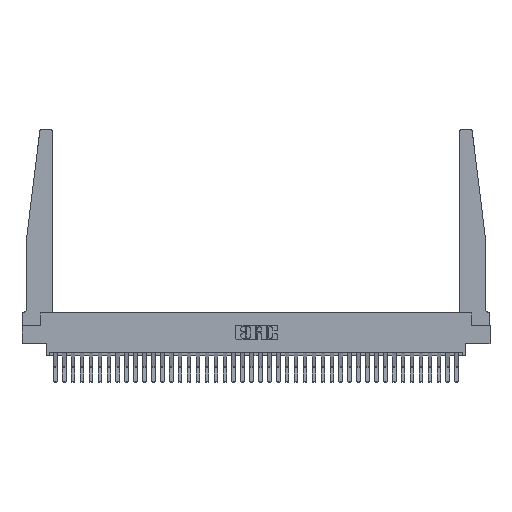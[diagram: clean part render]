
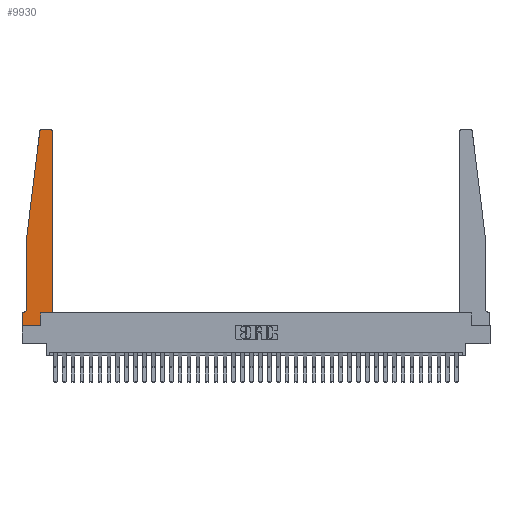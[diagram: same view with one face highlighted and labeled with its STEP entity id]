
A CAD part, top view. The second image highlights one B-rep face of the part: STEP entity #9930.
In plain terms, the highlighted planar face has unit normal (0, 0, 1).
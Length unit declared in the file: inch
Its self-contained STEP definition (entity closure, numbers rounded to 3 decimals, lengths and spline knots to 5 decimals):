
#721 = CARTESIAN_POINT ( 'NONE',  ( 0., 0., 0.37 ) ) ;
#744 = VECTOR ( 'NONE', #24177, 39.37008 ) ;
#1113 = CARTESIAN_POINT ( 'NONE',  ( 0.065, 1.25, 0.37 ) ) ;
#1154 = VERTEX_POINT ( 'NONE', #30985 ) ;
#1266 = AXIS2_PLACEMENT_3D ( 'NONE', #10810, #29415, #13551 ) ;
#1383 = VERTEX_POINT ( 'NONE', #18739 ) ;
#1935 = CARTESIAN_POINT ( 'NONE',  ( 0.425, 2.72, 0.37 ) ) ;
#2070 = CARTESIAN_POINT ( 'NONE',  ( 0.2605, 0.18, 0.37 ) ) ;
#2180 = LINE ( 'NONE', #16580, #28918 ) ;
#3547 = CARTESIAN_POINT ( 'NONE',  ( 0.065, 0.1875, 0.37 ) ) ;
#4044 = VERTEX_POINT ( 'NONE', #24911 ) ;
#4615 = LINE ( 'NONE', #6835, #32141 ) ;
#4649 = DIRECTION ( 'NONE',  ( 1., 0., 0. ) ) ;
#4755 = LINE ( 'NONE', #2070, #25186 ) ;
#4769 = VERTEX_POINT ( 'NONE', #19481 ) ;
#5407 = CARTESIAN_POINT ( 'NONE',  ( 0.425, 0.18, 0.37 ) ) ;
#5618 = VERTEX_POINT ( 'NONE', #15215 ) ;
#5651 = EDGE_CURVE ( 'NONE', #32344, #1383, #13668, .T. ) ;
#5811 = ORIENTED_EDGE ( 'NONE', *, *, #29186, .T. ) ;
#5827 = CARTESIAN_POINT ( 'NONE',  ( 0.395, 2.72, 0.37 ) ) ;
#5858 = LINE ( 'NONE', #1113, #20130 ) ;
#5941 = ORIENTED_EDGE ( 'NONE', *, *, #29677, .T. ) ;
#6488 = PLANE ( 'NONE',  #16297 ) ;
#6835 = CARTESIAN_POINT ( 'NONE',  ( 0.25, 2.75, 0.37 ) ) ;
#7605 = DIRECTION ( 'NONE',  ( 0., 1., 0. ) ) ;
#7629 = LINE ( 'NONE', #23846, #21863 ) ;
#7861 = DIRECTION ( 'NONE',  ( 0., -1., 0. ) ) ;
#8511 = DIRECTION ( 'NONE',  ( 1., 0., 0. ) ) ;
#9526 = DIRECTION ( 'NONE',  ( -1., 0., 0. ) ) ;
#9733 = EDGE_CURVE ( 'NONE', #33349, #13416, #17219, .T. ) ;
#9907 = EDGE_CURVE ( 'NONE', #10976, #4044, #5858, .T. ) ;
#9930 = ADVANCED_FACE ( 'NONE', ( #26295 ), #6488, .T. ) ;
#10309 = EDGE_CURVE ( 'NONE', #5618, #10976, #27094, .T. ) ;
#10810 = CARTESIAN_POINT ( 'NONE',  ( 0.015, 0.2375, 0.37 ) ) ;
#10934 = DIRECTION ( 'NONE',  ( 0., 0., 1. ) ) ;
#10976 = VERTEX_POINT ( 'NONE', #13622 ) ;
#10989 = EDGE_CURVE ( 'NONE', #27133, #33349, #29122, .T. ) ;
#11595 = VERTEX_POINT ( 'NONE', #19071 ) ;
#11765 = EDGE_CURVE ( 'NONE', #4769, #1154, #20833, .T. ) ;
#11831 = ORIENTED_EDGE ( 'NONE', *, *, #5651, .T. ) ;
#12662 = CARTESIAN_POINT ( 'NONE',  ( 0., 0., 0.37 ) ) ;
#12934 = LINE ( 'NONE', #33450, #27028 ) ;
#13416 = VERTEX_POINT ( 'NONE', #14213 ) ;
#13551 = DIRECTION ( 'NONE',  ( -1., 0., 0. ) ) ;
#13622 = CARTESIAN_POINT ( 'NONE',  ( 0.24675, 2.72367, 0.37 ) ) ;
#13668 = LINE ( 'NONE', #12662, #33142 ) ;
#13744 = EDGE_CURVE ( 'NONE', #1383, #11595, #4755, .T. ) ;
#13981 = ORIENTED_EDGE ( 'NONE', *, *, #10309, .T. ) ;
#14213 = CARTESIAN_POINT ( 'NONE',  ( 0.395, 2.75, 0.37 ) ) ;
#15215 = CARTESIAN_POINT ( 'NONE',  ( 0.27653, 2.75, 0.37 ) ) ;
#16213 = ORIENTED_EDGE ( 'NONE', *, *, #24653, .T. ) ;
#16259 = EDGE_CURVE ( 'NONE', #11595, #27133, #12934, .T. ) ;
#16287 = ORIENTED_EDGE ( 'NONE', *, *, #9907, .T. ) ;
#16297 = AXIS2_PLACEMENT_3D ( 'NONE', #25158, #33146, #17320 ) ;
#16580 = CARTESIAN_POINT ( 'NONE',  ( 0., 0., 0.37 ) ) ;
#17110 = CARTESIAN_POINT ( 'NONE',  ( 0.065, 0.2375, 0.37 ) ) ;
#17210 = DIRECTION ( 'NONE',  ( -0.122, -0.992, 0. ) ) ;
#17219 = CIRCLE ( 'NONE', #25814, 0.03 ) ;
#17320 = DIRECTION ( 'NONE',  ( 1., 0., 0. ) ) ;
#18739 = CARTESIAN_POINT ( 'NONE',  ( 0.2605, 0., 0.37 ) ) ;
#19071 = CARTESIAN_POINT ( 'NONE',  ( 0.2605, 0.18, 0.37 ) ) ;
#19149 = VECTOR ( 'NONE', #19640, 39.37008 ) ;
#19266 = DIRECTION ( 'NONE',  ( 0., -1., 0. ) ) ;
#19481 = CARTESIAN_POINT ( 'NONE',  ( 0.015, 0.1875, 0.37 ) ) ;
#19523 = ORIENTED_EDGE ( 'NONE', *, *, #16259, .T. ) ;
#19640 = DIRECTION ( 'NONE',  ( -1., 0., 0. ) ) ;
#20130 = VECTOR ( 'NONE', #17210, 39.37008 ) ;
#20298 = DIRECTION ( 'NONE',  ( 1., 0., 0. ) ) ;
#20590 = ORIENTED_EDGE ( 'NONE', *, *, #10989, .T. ) ;
#20833 = LINE ( 'NONE', #3547, #19149 ) ;
#21863 = VECTOR ( 'NONE', #7861, 39.37008 ) ;
#22524 = EDGE_CURVE ( 'NONE', #13416, #5618, #4615, .T. ) ;
#23846 = CARTESIAN_POINT ( 'NONE',  ( 0.065, 1.25, 0.37 ) ) ;
#24177 = DIRECTION ( 'NONE',  ( 0., 1., 0. ) ) ;
#24475 = DIRECTION ( 'NONE',  ( 0., 0., 1. ) ) ;
#24653 = EDGE_CURVE ( 'NONE', #31327, #4769, #32397, .T. ) ;
#24911 = CARTESIAN_POINT ( 'NONE',  ( 0.065, 1.25, 0.37 ) ) ;
#25158 = CARTESIAN_POINT ( 'NONE',  ( 0., 0.1875, 0.37 ) ) ;
#25186 = VECTOR ( 'NONE', #7605, 39.37008 ) ;
#25353 = ORIENTED_EDGE ( 'NONE', *, *, #22524, .T. ) ;
#25443 = ORIENTED_EDGE ( 'NONE', *, *, #9733, .T. ) ;
#25814 = AXIS2_PLACEMENT_3D ( 'NONE', #5827, #24475, #8511 ) ;
#26295 = FACE_OUTER_BOUND ( 'NONE', #31811, .T. ) ;
#26862 = CARTESIAN_POINT ( 'NONE',  ( 0.27653, 2.72, 0.37 ) ) ;
#27028 = VECTOR ( 'NONE', #20298, 39.37008 ) ;
#27094 = CIRCLE ( 'NONE', #29825, 0.03 ) ;
#27133 = VERTEX_POINT ( 'NONE', #5407 ) ;
#28101 = ORIENTED_EDGE ( 'NONE', *, *, #11765, .T. ) ;
#28918 = VECTOR ( 'NONE', #19266, 39.37008 ) ;
#29122 = LINE ( 'NONE', #29609, #744 ) ;
#29186 = EDGE_CURVE ( 'NONE', #1154, #32344, #2180, .T. ) ;
#29415 = DIRECTION ( 'NONE',  ( 0., 0., -1. ) ) ;
#29534 = DIRECTION ( 'NONE',  ( 1., 0., 0. ) ) ;
#29609 = CARTESIAN_POINT ( 'NONE',  ( 0.425, 0.18, 0.37 ) ) ;
#29677 = EDGE_CURVE ( 'NONE', #4044, #31327, #7629, .T. ) ;
#29825 = AXIS2_PLACEMENT_3D ( 'NONE', #26862, #10934, #29534 ) ;
#30985 = CARTESIAN_POINT ( 'NONE',  ( 0., 0.1875, 0.37 ) ) ;
#31327 = VERTEX_POINT ( 'NONE', #17110 ) ;
#31811 = EDGE_LOOP ( 'NONE', ( #25353, #13981, #16287, #5941, #16213, #28101, #5811, #11831, #32276, #19523, #20590, #25443 ) ) ;
#32141 = VECTOR ( 'NONE', #9526, 39.37008 ) ;
#32276 = ORIENTED_EDGE ( 'NONE', *, *, #13744, .T. ) ;
#32344 = VERTEX_POINT ( 'NONE', #721 ) ;
#32397 = CIRCLE ( 'NONE', #1266, 0.05 ) ;
#33142 = VECTOR ( 'NONE', #4649, 39.37008 ) ;
#33146 = DIRECTION ( 'NONE',  ( 0., 0., 1. ) ) ;
#33349 = VERTEX_POINT ( 'NONE', #1935 ) ;
#33450 = CARTESIAN_POINT ( 'NONE',  ( 0.425, 0.18, 0.37 ) ) ;
